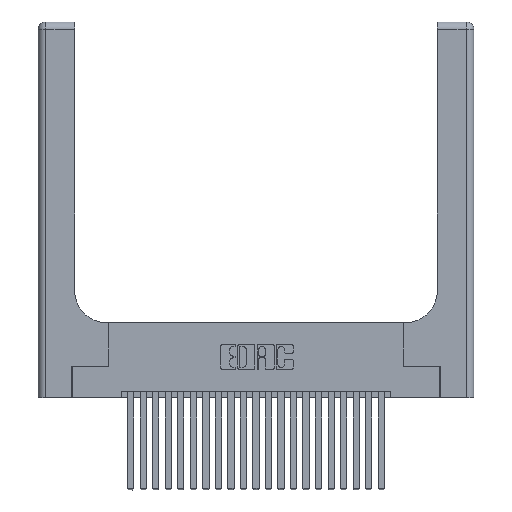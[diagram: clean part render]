
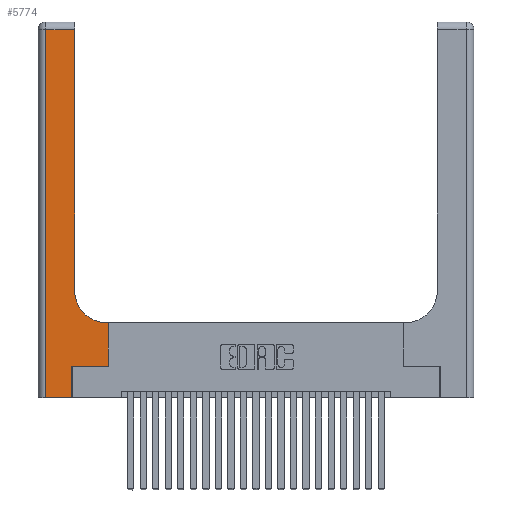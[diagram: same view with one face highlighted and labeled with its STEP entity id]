
A CAD part, top view. The second image highlights one B-rep face of the part: STEP entity #5774.
In plain terms, the highlighted planar face has unit normal (0, 0, 1).
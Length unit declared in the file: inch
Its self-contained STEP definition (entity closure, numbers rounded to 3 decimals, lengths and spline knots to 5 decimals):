
#175 = DIRECTION ( 'NONE',  ( 0., 1., 0. ) ) ;
#861 = VERTEX_POINT ( 'NONE', #20967 ) ;
#892 = CARTESIAN_POINT ( 'NONE',  ( 0.06, 2.94, 0.37 ) ) ;
#1255 = EDGE_LOOP ( 'NONE', ( #23495, #9727, #23311, #3544, #2789, #24222, #7424, #12704, #5242 ) ) ;
#1411 = VECTOR ( 'NONE', #5632, 39.37008 ) ;
#2789 = ORIENTED_EDGE ( 'NONE', *, *, #20028, .T. ) ;
#3344 = VERTEX_POINT ( 'NONE', #8568 ) ;
#3544 = ORIENTED_EDGE ( 'NONE', *, *, #22844, .T. ) ;
#3696 = EDGE_CURVE ( 'NONE', #22914, #24227, #20008, .T. ) ;
#3745 = VECTOR ( 'NONE', #21924, 39.37008 ) ;
#4645 = CARTESIAN_POINT ( 'NONE',  ( 0.5415, 0.85, 0.37 ) ) ;
#5150 = VERTEX_POINT ( 'NONE', #16979 ) ;
#5188 = CARTESIAN_POINT ( 'NONE',  ( 0.2915, 3., 0.37 ) ) ;
#5242 = ORIENTED_EDGE ( 'NONE', *, *, #19657, .T. ) ;
#5310 = VECTOR ( 'NONE', #14468, 39.37008 ) ;
#5584 = LINE ( 'NONE', #11293, #10012 ) ;
#5632 = DIRECTION ( 'NONE',  ( 1., 0., 0. ) ) ;
#5664 = EDGE_CURVE ( 'NONE', #6172, #22914, #13149, .T. ) ;
#5774 = ADVANCED_FACE ( 'NONE', ( #6962 ), #10688, .F. ) ;
#6172 = VERTEX_POINT ( 'NONE', #17860 ) ;
#6962 = FACE_OUTER_BOUND ( 'NONE', #1255, .T. ) ;
#6995 = EDGE_CURVE ( 'NONE', #9177, #861, #16053, .T. ) ;
#7424 = ORIENTED_EDGE ( 'NONE', *, *, #13616, .T. ) ;
#7447 = CARTESIAN_POINT ( 'NONE',  ( 0., 0., 0.37 ) ) ;
#8515 = DIRECTION ( 'NONE',  ( 0., 0., -1. ) ) ;
#8518 = CARTESIAN_POINT ( 'NONE',  ( 0.06, 3., 0.37 ) ) ;
#8568 = CARTESIAN_POINT ( 'NONE',  ( 0.06, 0., 0.37 ) ) ;
#8587 = CARTESIAN_POINT ( 'NONE',  ( 0.5415, 0.6, 0.37 ) ) ;
#8861 = VECTOR ( 'NONE', #175, 39.37008 ) ;
#9177 = VERTEX_POINT ( 'NONE', #14657 ) ;
#9646 = CARTESIAN_POINT ( 'NONE',  ( 0.269, 0., 0.37 ) ) ;
#9722 = CARTESIAN_POINT ( 'NONE',  ( 0.269, 0., 0.37 ) ) ;
#9727 = ORIENTED_EDGE ( 'NONE', *, *, #3696, .T. ) ;
#9899 = DIRECTION ( 'NONE',  ( -1., 0., 0. ) ) ;
#9968 = VECTOR ( 'NONE', #24032, 39.37008 ) ;
#10004 = LINE ( 'NONE', #8518, #23798 ) ;
#10012 = VECTOR ( 'NONE', #13173, 39.37008 ) ;
#10688 = PLANE ( 'NONE',  #19425 ) ;
#10941 = CARTESIAN_POINT ( 'NONE',  ( 0.269, 0.25, 0.37 ) ) ;
#11149 = DIRECTION ( 'NONE',  ( 0., 0., -1. ) ) ;
#11293 = CARTESIAN_POINT ( 'NONE',  ( 0.2915, 0.6, 0.37 ) ) ;
#11695 = LINE ( 'NONE', #7447, #1411 ) ;
#12130 = CIRCLE ( 'NONE', #22620, 0.25 ) ;
#12341 = EDGE_CURVE ( 'NONE', #5150, #23257, #5584, .T. ) ;
#12415 = LINE ( 'NONE', #9646, #8861 ) ;
#12631 = CARTESIAN_POINT ( 'NONE',  ( 0., 3., 0.37 ) ) ;
#12704 = ORIENTED_EDGE ( 'NONE', *, *, #12341, .T. ) ;
#12812 = DIRECTION ( 'NONE',  ( 1., 0., 0. ) ) ;
#13149 = LINE ( 'NONE', #5188, #3745 ) ;
#13173 = DIRECTION ( 'NONE',  ( -1., 0., 0. ) ) ;
#13616 = EDGE_CURVE ( 'NONE', #861, #5150, #17618, .T. ) ;
#14447 = DIRECTION ( 'NONE',  ( 0., -1., 0. ) ) ;
#14468 = DIRECTION ( 'NONE',  ( -1., 0., 0. ) ) ;
#14657 = CARTESIAN_POINT ( 'NONE',  ( 0.269, 0.25, 0.37 ) ) ;
#16053 = LINE ( 'NONE', #10941, #18673 ) ;
#16843 = CARTESIAN_POINT ( 'NONE',  ( 0.5585, 0.25, 0.37 ) ) ;
#16979 = CARTESIAN_POINT ( 'NONE',  ( 0.5585, 0.6, 0.37 ) ) ;
#17618 = LINE ( 'NONE', #16843, #9968 ) ;
#17860 = CARTESIAN_POINT ( 'NONE',  ( 0.2915, 0.85, 0.37 ) ) ;
#18673 = VECTOR ( 'NONE', #12812, 39.37008 ) ;
#19425 = AXIS2_PLACEMENT_3D ( 'NONE', #12631, #11149, #9899 ) ;
#19657 = EDGE_CURVE ( 'NONE', #23257, #6172, #12130, .T. ) ;
#20008 = LINE ( 'NONE', #20032, #5310 ) ;
#20024 = VERTEX_POINT ( 'NONE', #9722 ) ;
#20028 = EDGE_CURVE ( 'NONE', #20024, #9177, #12415, .T. ) ;
#20032 = CARTESIAN_POINT ( 'NONE',  ( 0., 2.94, 0.37 ) ) ;
#20967 = CARTESIAN_POINT ( 'NONE',  ( 0.5585, 0.25, 0.37 ) ) ;
#21508 = EDGE_CURVE ( 'NONE', #24227, #3344, #10004, .T. ) ;
#21618 = DIRECTION ( 'NONE',  ( 1., 0., 0. ) ) ;
#21924 = DIRECTION ( 'NONE',  ( 0., 1., 0. ) ) ;
#22434 = CARTESIAN_POINT ( 'NONE',  ( 0.2915, 2.94, 0.37 ) ) ;
#22620 = AXIS2_PLACEMENT_3D ( 'NONE', #4645, #8515, #21618 ) ;
#22844 = EDGE_CURVE ( 'NONE', #3344, #20024, #11695, .T. ) ;
#22914 = VERTEX_POINT ( 'NONE', #22434 ) ;
#23257 = VERTEX_POINT ( 'NONE', #8587 ) ;
#23311 = ORIENTED_EDGE ( 'NONE', *, *, #21508, .T. ) ;
#23495 = ORIENTED_EDGE ( 'NONE', *, *, #5664, .T. ) ;
#23798 = VECTOR ( 'NONE', #14447, 39.37008 ) ;
#24032 = DIRECTION ( 'NONE',  ( 0., 1., 0. ) ) ;
#24222 = ORIENTED_EDGE ( 'NONE', *, *, #6995, .T. ) ;
#24227 = VERTEX_POINT ( 'NONE', #892 ) ;
